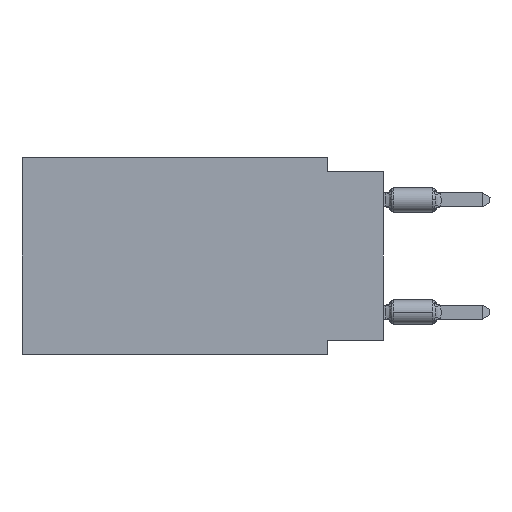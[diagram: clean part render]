
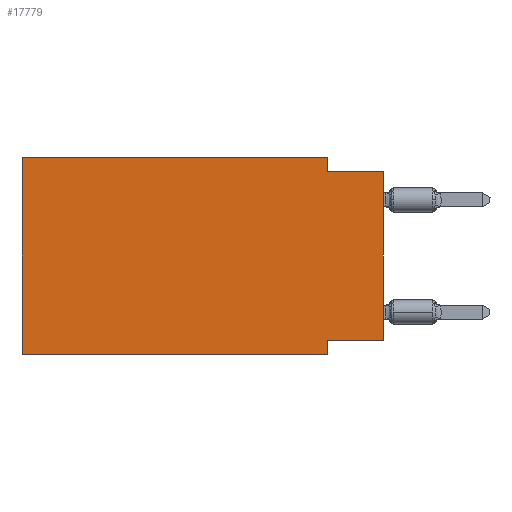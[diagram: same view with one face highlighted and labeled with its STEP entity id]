
A CAD part, left-side view. The second image highlights one B-rep face of the part: STEP entity #17779.
In plain terms, the highlighted planar face has unit normal (-1, 0, 0).
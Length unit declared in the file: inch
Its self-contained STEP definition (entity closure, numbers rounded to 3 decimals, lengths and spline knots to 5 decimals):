
#420 = CARTESIAN_POINT ( 'NONE',  ( 0., 0.645, 0. ) ) ;
#1415 = CARTESIAN_POINT ( 'NONE',  ( 0., 0.645, 0. ) ) ;
#1599 = VECTOR ( 'NONE', #6670, 39.37008 ) ;
#2400 = EDGE_LOOP ( 'NONE', ( #32236, #49120, #17778, #13564, #7993, #4857, #32028, #12726 ) ) ;
#2542 = VECTOR ( 'NONE', #59250, 39.37008 ) ;
#3238 = DIRECTION ( 'NONE',  ( 0., 0., 1. ) ) ;
#3602 = VERTEX_POINT ( 'NONE', #35717 ) ;
#3888 = EDGE_CURVE ( 'NONE', #55999, #19252, #49675, .T. ) ;
#3941 = VECTOR ( 'NONE', #32047, 39.37008 ) ;
#4857 = ORIENTED_EDGE ( 'NONE', *, *, #54455, .T. ) ;
#6160 = DIRECTION ( 'NONE',  ( 0., 0., -1. ) ) ;
#6670 = DIRECTION ( 'NONE',  ( 0., -1., 0. ) ) ;
#6801 = DIRECTION ( 'NONE',  ( 0., 0., 1. ) ) ;
#7028 = VECTOR ( 'NONE', #8082, 39.37008 ) ;
#7760 = CARTESIAN_POINT ( 'NONE',  ( 0., 0., 0. ) ) ;
#7993 = ORIENTED_EDGE ( 'NONE', *, *, #32704, .F. ) ;
#8082 = DIRECTION ( 'NONE',  ( 0., 1., 0. ) ) ;
#8192 = CARTESIAN_POINT ( 'NONE',  ( 0., 0.645, 0. ) ) ;
#9033 = VERTEX_POINT ( 'NONE', #52925 ) ;
#9039 = CARTESIAN_POINT ( 'NONE',  ( 0., 0.645, -0.35 ) ) ;
#11304 = LINE ( 'NONE', #1415, #26064 ) ;
#12726 = ORIENTED_EDGE ( 'NONE', *, *, #26673, .F. ) ;
#13564 = ORIENTED_EDGE ( 'NONE', *, *, #3888, .F. ) ;
#14528 = EDGE_CURVE ( 'NONE', #9033, #26897, #17035, .T. ) ;
#15036 = CARTESIAN_POINT ( 'NONE',  ( 0., 0.1, -0.025 ) ) ;
#15105 = CARTESIAN_POINT ( 'NONE',  ( 0., 0., -0.025 ) ) ;
#15286 = VECTOR ( 'NONE', #3238, 39.37008 ) ;
#15358 = CARTESIAN_POINT ( 'NONE',  ( 0., 0., -0.325 ) ) ;
#17035 = LINE ( 'NONE', #59122, #3941 ) ;
#17778 = ORIENTED_EDGE ( 'NONE', *, *, #49487, .F. ) ;
#17779 = ADVANCED_FACE ( 'NONE', ( #24207 ), #19690, .F. ) ;
#18534 = VERTEX_POINT ( 'NONE', #15036 ) ;
#19098 = CARTESIAN_POINT ( 'NONE',  ( 0., 0.645, 0. ) ) ;
#19252 = VERTEX_POINT ( 'NONE', #44383 ) ;
#19690 = PLANE ( 'NONE',  #53204 ) ;
#21739 = LINE ( 'NONE', #39776, #44174 ) ;
#24207 = FACE_OUTER_BOUND ( 'NONE', #2400, .T. ) ;
#24283 = EDGE_CURVE ( 'NONE', #18534, #3602, #47853, .T. ) ;
#24871 = CARTESIAN_POINT ( 'NONE',  ( 0., 0.1, -0.35 ) ) ;
#25805 = LINE ( 'NONE', #7760, #15286 ) ;
#26064 = VECTOR ( 'NONE', #6801, 39.37008 ) ;
#26673 = EDGE_CURVE ( 'NONE', #51084, #9033, #48967, .T. ) ;
#26714 = CARTESIAN_POINT ( 'NONE',  ( 0., 0., -0.325 ) ) ;
#26847 = CARTESIAN_POINT ( 'NONE',  ( 0., 0.645, -0.35 ) ) ;
#26897 = VERTEX_POINT ( 'NONE', #24871 ) ;
#32028 = ORIENTED_EDGE ( 'NONE', *, *, #14528, .F. ) ;
#32047 = DIRECTION ( 'NONE',  ( 0., 0., -1. ) ) ;
#32236 = ORIENTED_EDGE ( 'NONE', *, *, #48570, .T. ) ;
#32704 = EDGE_CURVE ( 'NONE', #45020, #55999, #11304, .T. ) ;
#35717 = CARTESIAN_POINT ( 'NONE',  ( 0., 0., -0.025 ) ) ;
#35832 = DIRECTION ( 'NONE',  ( 0., -1., 0. ) ) ;
#38030 = DIRECTION ( 'NONE',  ( 1., 0., 0. ) ) ;
#39776 = CARTESIAN_POINT ( 'NONE',  ( 0., 0.1, 0. ) ) ;
#44174 = VECTOR ( 'NONE', #58118, 39.37008 ) ;
#44383 = CARTESIAN_POINT ( 'NONE',  ( 0., 0.1, 0. ) ) ;
#45020 = VERTEX_POINT ( 'NONE', #26847 ) ;
#47853 = LINE ( 'NONE', #15105, #1599 ) ;
#48570 = EDGE_CURVE ( 'NONE', #51084, #3602, #25805, .T. ) ;
#48967 = LINE ( 'NONE', #26714, #7028 ) ;
#49120 = ORIENTED_EDGE ( 'NONE', *, *, #24283, .F. ) ;
#49487 = EDGE_CURVE ( 'NONE', #19252, #18534, #21739, .T. ) ;
#49675 = LINE ( 'NONE', #8192, #50422 ) ;
#50422 = VECTOR ( 'NONE', #35832, 39.37008 ) ;
#50527 = LINE ( 'NONE', #9039, #2542 ) ;
#51084 = VERTEX_POINT ( 'NONE', #15358 ) ;
#52925 = CARTESIAN_POINT ( 'NONE',  ( 0., 0.1, -0.325 ) ) ;
#53204 = AXIS2_PLACEMENT_3D ( 'NONE', #19098, #38030, #6160 ) ;
#54455 = EDGE_CURVE ( 'NONE', #45020, #26897, #50527, .T. ) ;
#55999 = VERTEX_POINT ( 'NONE', #420 ) ;
#58118 = DIRECTION ( 'NONE',  ( 0., 0., -1. ) ) ;
#59122 = CARTESIAN_POINT ( 'NONE',  ( 0., 0.1, -0.35 ) ) ;
#59250 = DIRECTION ( 'NONE',  ( 0., -1., 0. ) ) ;
